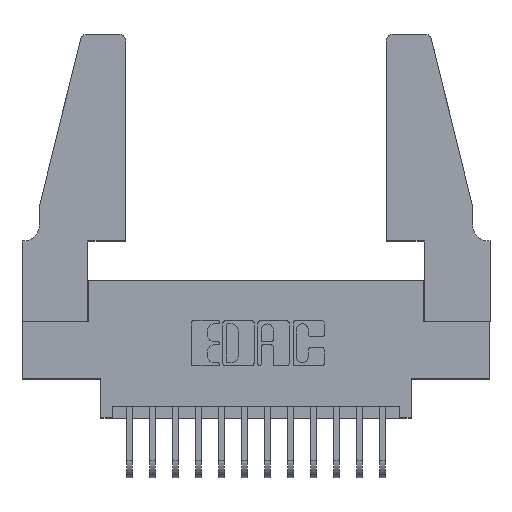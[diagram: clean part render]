
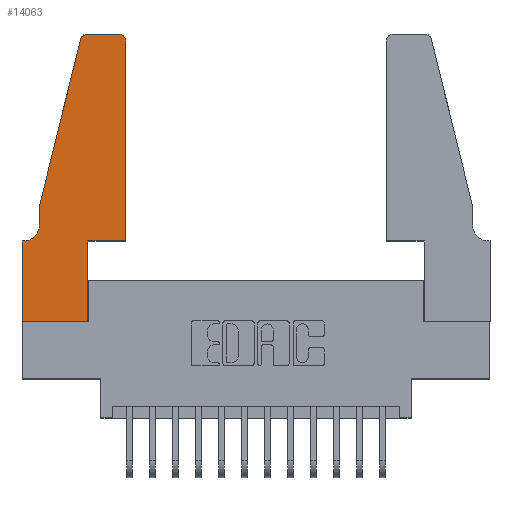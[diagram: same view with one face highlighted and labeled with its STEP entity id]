
A CAD part, top view. The second image highlights one B-rep face of the part: STEP entity #14063.
In plain terms, the highlighted planar face has unit normal (0, 0, 1).
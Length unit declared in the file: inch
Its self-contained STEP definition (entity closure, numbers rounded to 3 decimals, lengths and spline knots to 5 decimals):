
#60 = VERTEX_POINT ( 'NONE', #6562 ) ;
#118 = VERTEX_POINT ( 'NONE', #11315 ) ;
#268 = ORIENTED_EDGE ( 'NONE', *, *, #6899, .T. ) ;
#364 = AXIS2_PLACEMENT_3D ( 'NONE', #17132, #15849, #13167 ) ;
#405 = EDGE_CURVE ( 'NONE', #118, #11470, #580, .T. ) ;
#502 = DIRECTION ( 'NONE',  ( 1., 0., 0. ) ) ;
#526 = VECTOR ( 'NONE', #5932, 39.37008 ) ;
#544 = VERTEX_POINT ( 'NONE', #1698 ) ;
#580 = LINE ( 'NONE', #2344, #17208 ) ;
#1071 = EDGE_CURVE ( 'NONE', #3733, #118, #4096, .T. ) ;
#1287 = LINE ( 'NONE', #9212, #13524 ) ;
#1698 = CARTESIAN_POINT ( 'NONE',  ( 0.0055, 0.35, 0.37 ) ) ;
#1886 = DIRECTION ( 'NONE',  ( 0., 1., 0. ) ) ;
#1962 = LINE ( 'NONE', #6169, #9591 ) ;
#2344 = CARTESIAN_POINT ( 'NONE',  ( 0.2605, 1.25, 0.37 ) ) ;
#2464 = ORIENTED_EDGE ( 'NONE', *, *, #2862, .T. ) ;
#2491 = CARTESIAN_POINT ( 'NONE',  ( 0.2865, 0., 0.37 ) ) ;
#2625 = DIRECTION ( 'NONE',  ( 0., 0., 1. ) ) ;
#2675 = DIRECTION ( 'NONE',  ( 1., 0., 0. ) ) ;
#2749 = DIRECTION ( 'NONE',  ( 1., 0., 0. ) ) ;
#2795 = CARTESIAN_POINT ( 'NONE',  ( 0.0755, 0.5, 0.37 ) ) ;
#2862 = EDGE_CURVE ( 'NONE', #8579, #11004, #4066, .T. ) ;
#3142 = ORIENTED_EDGE ( 'NONE', *, *, #9259, .T. ) ;
#3318 = EDGE_CURVE ( 'NONE', #6330, #13285, #5327, .T. ) ;
#3441 = ORIENTED_EDGE ( 'NONE', *, *, #3318, .T. ) ;
#3616 = LINE ( 'NONE', #9462, #8514 ) ;
#3733 = VERTEX_POINT ( 'NONE', #13302 ) ;
#4028 = FACE_OUTER_BOUND ( 'NONE', #6095, .T. ) ;
#4066 = LINE ( 'NONE', #8498, #526 ) ;
#4096 = CIRCLE ( 'NONE', #10711, 0.03 ) ;
#4293 = CARTESIAN_POINT ( 'NONE',  ( 0.2865, 0.35, 0.37 ) ) ;
#4376 = EDGE_CURVE ( 'NONE', #4499, #11240, #1287, .T. ) ;
#4499 = VERTEX_POINT ( 'NONE', #17190 ) ;
#5037 = DIRECTION ( 'NONE',  ( -1., 0., 0. ) ) ;
#5214 = VECTOR ( 'NONE', #6661, 39.37008 ) ;
#5327 = LINE ( 'NONE', #11120, #13155 ) ;
#5341 = CARTESIAN_POINT ( 'NONE',  ( 0.0755, 0.35, 0.37 ) ) ;
#5368 = LINE ( 'NONE', #15042, #12142 ) ;
#5932 = DIRECTION ( 'NONE',  ( 0., -1., 0. ) ) ;
#6095 = EDGE_LOOP ( 'NONE', ( #13746, #11723, #10170, #16801, #17081, #268, #2464, #6791, #3441, #3142, #14400, #12058 ) ) ;
#6169 = CARTESIAN_POINT ( 'NONE',  ( 0.4505, 0.35, 0.37 ) ) ;
#6330 = VERTEX_POINT ( 'NONE', #2491 ) ;
#6562 = CARTESIAN_POINT ( 'NONE',  ( 0.4505, 0.35, 0.37 ) ) ;
#6616 = CARTESIAN_POINT ( 'NONE',  ( 0.0055, 0.42, 0.37 ) ) ;
#6661 = DIRECTION ( 'NONE',  ( -1., 0., 0. ) ) ;
#6791 = ORIENTED_EDGE ( 'NONE', *, *, #8430, .T. ) ;
#6899 = EDGE_CURVE ( 'NONE', #544, #8579, #8807, .T. ) ;
#7832 = CARTESIAN_POINT ( 'NONE',  ( 0., 0., 0.37 ) ) ;
#7874 = LINE ( 'NONE', #2795, #15431 ) ;
#8313 = DIRECTION ( 'NONE',  ( 1., 0., 0. ) ) ;
#8430 = EDGE_CURVE ( 'NONE', #11004, #6330, #5368, .T. ) ;
#8498 = CARTESIAN_POINT ( 'NONE',  ( 0., 0., 0.37 ) ) ;
#8514 = VECTOR ( 'NONE', #2749, 39.37008 ) ;
#8530 = EDGE_CURVE ( 'NONE', #60, #3733, #1962, .T. ) ;
#8579 = VERTEX_POINT ( 'NONE', #9252 ) ;
#8807 = LINE ( 'NONE', #5341, #5214 ) ;
#9101 = CIRCLE ( 'NONE', #12644, 0.03 ) ;
#9212 = CARTESIAN_POINT ( 'NONE',  ( 0.0755, 0.5, 0.37 ) ) ;
#9252 = CARTESIAN_POINT ( 'NONE',  ( 0., 0.35, 0.37 ) ) ;
#9259 = EDGE_CURVE ( 'NONE', #13285, #60, #3616, .T. ) ;
#9462 = CARTESIAN_POINT ( 'NONE',  ( 0.4505, 0.35, 0.37 ) ) ;
#9580 = CARTESIAN_POINT ( 'NONE',  ( 0.4205, 1.22, 0.37 ) ) ;
#9591 = VECTOR ( 'NONE', #11971, 39.37008 ) ;
#10147 = EDGE_CURVE ( 'NONE', #11240, #15321, #7874, .T. ) ;
#10170 = ORIENTED_EDGE ( 'NONE', *, *, #4376, .T. ) ;
#10345 = CIRCLE ( 'NONE', #16996, 0.07 ) ;
#10679 = DIRECTION ( 'NONE',  ( -1., 0., 0. ) ) ;
#10711 = AXIS2_PLACEMENT_3D ( 'NONE', #9580, #2625, #2675 ) ;
#10788 = CARTESIAN_POINT ( 'NONE',  ( 0.0755, 0.5, 0.37 ) ) ;
#10905 = EDGE_CURVE ( 'NONE', #11470, #4499, #9101, .T. ) ;
#11004 = VERTEX_POINT ( 'NONE', #7832 ) ;
#11120 = CARTESIAN_POINT ( 'NONE',  ( 0.2865, 0.35, 0.37 ) ) ;
#11240 = VERTEX_POINT ( 'NONE', #10788 ) ;
#11283 = EDGE_CURVE ( 'NONE', #15321, #544, #10345, .T. ) ;
#11315 = CARTESIAN_POINT ( 'NONE',  ( 0.4205, 1.25, 0.37 ) ) ;
#11470 = VERTEX_POINT ( 'NONE', #12797 ) ;
#11723 = ORIENTED_EDGE ( 'NONE', *, *, #10905, .T. ) ;
#11971 = DIRECTION ( 'NONE',  ( 0., 1., 0. ) ) ;
#12058 = ORIENTED_EDGE ( 'NONE', *, *, #1071, .T. ) ;
#12142 = VECTOR ( 'NONE', #502, 39.37008 ) ;
#12644 = AXIS2_PLACEMENT_3D ( 'NONE', #16428, #14837, #8313 ) ;
#12797 = CARTESIAN_POINT ( 'NONE',  ( 0.284, 1.25, 0.37 ) ) ;
#13043 = DIRECTION ( 'NONE',  ( -0.239, -0.971, 0. ) ) ;
#13155 = VECTOR ( 'NONE', #1886, 39.37008 ) ;
#13167 = DIRECTION ( 'NONE',  ( 1., 0., 0. ) ) ;
#13285 = VERTEX_POINT ( 'NONE', #4293 ) ;
#13302 = CARTESIAN_POINT ( 'NONE',  ( 0.4505, 1.22, 0.37 ) ) ;
#13524 = VECTOR ( 'NONE', #13043, 39.37008 ) ;
#13746 = ORIENTED_EDGE ( 'NONE', *, *, #405, .T. ) ;
#14063 = ADVANCED_FACE ( 'NONE', ( #4028 ), #15907, .T. ) ;
#14400 = ORIENTED_EDGE ( 'NONE', *, *, #8530, .T. ) ;
#14837 = DIRECTION ( 'NONE',  ( 0., 0., 1. ) ) ;
#15042 = CARTESIAN_POINT ( 'NONE',  ( 0., 0., 0.37 ) ) ;
#15321 = VERTEX_POINT ( 'NONE', #15452 ) ;
#15431 = VECTOR ( 'NONE', #17430, 39.37008 ) ;
#15452 = CARTESIAN_POINT ( 'NONE',  ( 0.0755, 0.42, 0.37 ) ) ;
#15849 = DIRECTION ( 'NONE',  ( 0., 0., 1. ) ) ;
#15907 = PLANE ( 'NONE',  #364 ) ;
#15959 = DIRECTION ( 'NONE',  ( 0., 0., -1. ) ) ;
#16428 = CARTESIAN_POINT ( 'NONE',  ( 0.284, 1.22, 0.37 ) ) ;
#16801 = ORIENTED_EDGE ( 'NONE', *, *, #10147, .T. ) ;
#16996 = AXIS2_PLACEMENT_3D ( 'NONE', #6616, #15959, #10679 ) ;
#17081 = ORIENTED_EDGE ( 'NONE', *, *, #11283, .T. ) ;
#17132 = CARTESIAN_POINT ( 'NONE',  ( 0., 0.35, 0.37 ) ) ;
#17190 = CARTESIAN_POINT ( 'NONE',  ( 0.25487, 1.22718, 0.37 ) ) ;
#17208 = VECTOR ( 'NONE', #5037, 39.37008 ) ;
#17430 = DIRECTION ( 'NONE',  ( 0., -1., 0. ) ) ;
